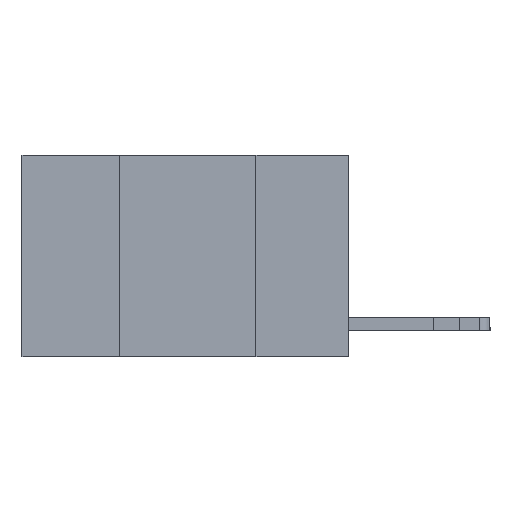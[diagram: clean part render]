
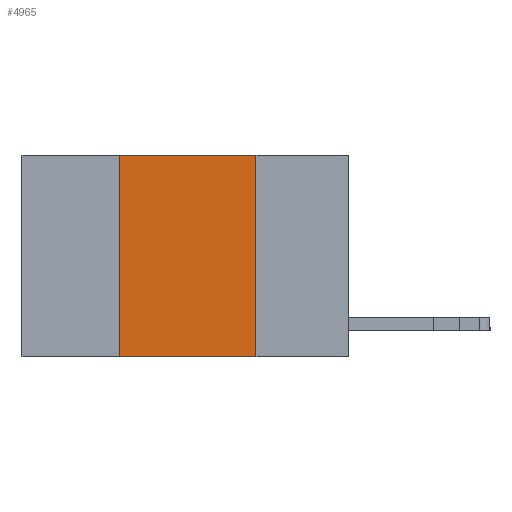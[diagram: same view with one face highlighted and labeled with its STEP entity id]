
A CAD part, left-side view. The second image highlights one B-rep face of the part: STEP entity #4965.
In plain terms, the highlighted planar face has unit normal (-1, 0, 0).
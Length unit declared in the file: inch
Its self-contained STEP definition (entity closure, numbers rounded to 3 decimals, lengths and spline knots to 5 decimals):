
#707 = EDGE_CURVE ( 'NONE', #6526, #722, #9866, .T. ) ;
#722 = VERTEX_POINT ( 'NONE', #2121 ) ;
#782 = CARTESIAN_POINT ( 'NONE',  ( 0., 0.6, 0. ) ) ;
#1928 = ORIENTED_EDGE ( 'NONE', *, *, #2459, .F. ) ;
#2037 = CARTESIAN_POINT ( 'NONE',  ( 0., 0.17, -0.37 ) ) ;
#2121 = CARTESIAN_POINT ( 'NONE',  ( 0., 0.17, 0. ) ) ;
#2144 = VERTEX_POINT ( 'NONE', #2037 ) ;
#2459 = EDGE_CURVE ( 'NONE', #3967, #6526, #4425, .T. ) ;
#2611 = DIRECTION ( 'NONE',  ( 0., 0., 1. ) ) ;
#3464 = EDGE_LOOP ( 'NONE', ( #9968, #7972, #1928, #11527 ) ) ;
#3921 = CARTESIAN_POINT ( 'NONE',  ( 0., 0.17, 0. ) ) ;
#3967 = VERTEX_POINT ( 'NONE', #11223 ) ;
#4147 = AXIS2_PLACEMENT_3D ( 'NONE', #11083, #6621, #10213 ) ;
#4425 = LINE ( 'NONE', #6999, #11227 ) ;
#4965 = ADVANCED_FACE ( 'NONE', ( #7496 ), #6678, .F. ) ;
#5863 = CARTESIAN_POINT ( 'NONE',  ( 0., 0.42, 0. ) ) ;
#6494 = EDGE_CURVE ( 'NONE', #3967, #2144, #8629, .T. ) ;
#6526 = VERTEX_POINT ( 'NONE', #5863 ) ;
#6621 = DIRECTION ( 'NONE',  ( 1., 0., 0. ) ) ;
#6678 = PLANE ( 'NONE',  #4147 ) ;
#6764 = VECTOR ( 'NONE', #8451, 39.37008 ) ;
#6970 = EDGE_CURVE ( 'NONE', #722, #2144, #11076, .T. ) ;
#6999 = CARTESIAN_POINT ( 'NONE',  ( 0., 0.42, 0. ) ) ;
#7144 = DIRECTION ( 'NONE',  ( 0., -1., 0. ) ) ;
#7496 = FACE_OUTER_BOUND ( 'NONE', #3464, .T. ) ;
#7972 = ORIENTED_EDGE ( 'NONE', *, *, #707, .F. ) ;
#8451 = DIRECTION ( 'NONE',  ( 0., -1., 0. ) ) ;
#8629 = LINE ( 'NONE', #11262, #6764 ) ;
#9028 = VECTOR ( 'NONE', #11017, 39.37008 ) ;
#9866 = LINE ( 'NONE', #782, #10494 ) ;
#9968 = ORIENTED_EDGE ( 'NONE', *, *, #6970, .F. ) ;
#10213 = DIRECTION ( 'NONE',  ( 0., 0., -1. ) ) ;
#10494 = VECTOR ( 'NONE', #7144, 39.37008 ) ;
#11017 = DIRECTION ( 'NONE',  ( 0., 0., -1. ) ) ;
#11076 = LINE ( 'NONE', #3921, #9028 ) ;
#11083 = CARTESIAN_POINT ( 'NONE',  ( 0., 0.6, 0. ) ) ;
#11223 = CARTESIAN_POINT ( 'NONE',  ( 0., 0.42, -0.37 ) ) ;
#11227 = VECTOR ( 'NONE', #2611, 39.37008 ) ;
#11262 = CARTESIAN_POINT ( 'NONE',  ( 0., 0.6, -0.37 ) ) ;
#11527 = ORIENTED_EDGE ( 'NONE', *, *, #6494, .T. ) ;
